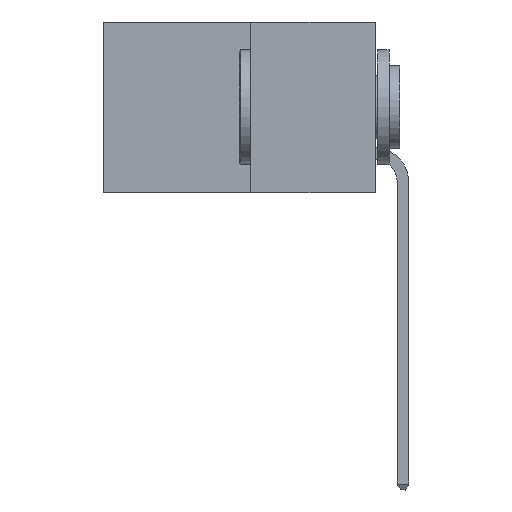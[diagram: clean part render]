
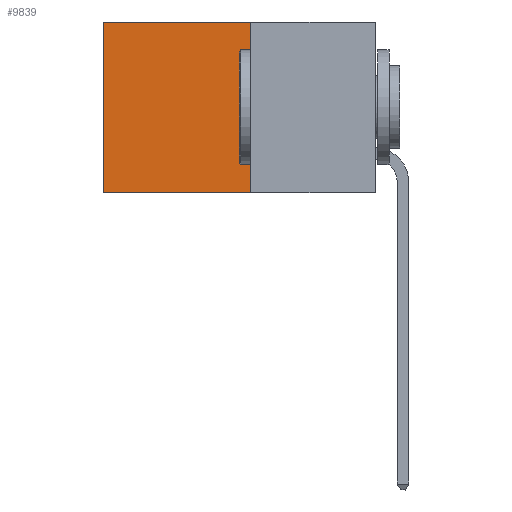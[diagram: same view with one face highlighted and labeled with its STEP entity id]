
A CAD part, left-side view. The second image highlights one B-rep face of the part: STEP entity #9839.
In plain terms, the highlighted planar face has unit normal (-1, 0, 0).
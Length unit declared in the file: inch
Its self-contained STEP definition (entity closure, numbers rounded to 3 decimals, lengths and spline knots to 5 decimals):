
#1183 = VERTEX_POINT ( 'NONE', #14891 ) ;
#7440 = CARTESIAN_POINT ( 'NONE',  ( 0.277, 0.27, 0. ) ) ;
#7531 = DIRECTION ( 'NONE',  ( 0., 1., 0. ) ) ;
#8829 = LINE ( 'NONE', #8898, #19447 ) ;
#8898 = CARTESIAN_POINT ( 'NONE',  ( 0.277, 0.59, -0.37 ) ) ;
#9678 = ORIENTED_EDGE ( 'NONE', *, *, #10059, .F. ) ;
#9839 = ADVANCED_FACE ( 'NONE', ( #27008 ), #12012, .F. ) ;
#9969 = CARTESIAN_POINT ( 'NONE',  ( 0.277, 0.27, -0.37 ) ) ;
#10059 = EDGE_CURVE ( 'NONE', #13811, #11825, #21227, .T. ) ;
#11825 = VERTEX_POINT ( 'NONE', #22484 ) ;
#12012 = PLANE ( 'NONE',  #18712 ) ;
#12119 = DIRECTION ( 'NONE',  ( 0., 1., 0. ) ) ;
#13300 = CARTESIAN_POINT ( 'NONE',  ( 0.277, 0.27, 0. ) ) ;
#13811 = VERTEX_POINT ( 'NONE', #13300 ) ;
#14052 = VECTOR ( 'NONE', #7531, 39.37008 ) ;
#14156 = LINE ( 'NONE', #9969, #25283 ) ;
#14185 = DIRECTION ( 'NONE',  ( 0., 0., -1. ) ) ;
#14630 = EDGE_CURVE ( 'NONE', #11825, #1183, #14156, .T. ) ;
#14891 = CARTESIAN_POINT ( 'NONE',  ( 0.277, 0.59, -0.37 ) ) ;
#15613 = VECTOR ( 'NONE', #23288, 39.37008 ) ;
#16370 = EDGE_CURVE ( 'NONE', #13811, #25216, #24551, .T. ) ;
#18712 = AXIS2_PLACEMENT_3D ( 'NONE', #24642, #26665, #14185 ) ;
#19447 = VECTOR ( 'NONE', #21589, 39.37008 ) ;
#19501 = EDGE_CURVE ( 'NONE', #25216, #1183, #8829, .T. ) ;
#21168 = CARTESIAN_POINT ( 'NONE',  ( 0.277, 0.27, -0.37 ) ) ;
#21227 = LINE ( 'NONE', #21168, #15613 ) ;
#21589 = DIRECTION ( 'NONE',  ( 0., 0., -1. ) ) ;
#22177 = ORIENTED_EDGE ( 'NONE', *, *, #16370, .T. ) ;
#22484 = CARTESIAN_POINT ( 'NONE',  ( 0.277, 0.27, -0.37 ) ) ;
#23288 = DIRECTION ( 'NONE',  ( 0., 0., -1. ) ) ;
#23738 = ORIENTED_EDGE ( 'NONE', *, *, #19501, .T. ) ;
#23976 = CARTESIAN_POINT ( 'NONE',  ( 0.277, 0.59, 0. ) ) ;
#24497 = EDGE_LOOP ( 'NONE', ( #23738, #26835, #9678, #22177 ) ) ;
#24551 = LINE ( 'NONE', #7440, #14052 ) ;
#24642 = CARTESIAN_POINT ( 'NONE',  ( 0.277, 0.27, -0.37 ) ) ;
#25216 = VERTEX_POINT ( 'NONE', #23976 ) ;
#25283 = VECTOR ( 'NONE', #12119, 39.37008 ) ;
#26665 = DIRECTION ( 'NONE',  ( 1., 0., 0. ) ) ;
#26835 = ORIENTED_EDGE ( 'NONE', *, *, #14630, .F. ) ;
#27008 = FACE_OUTER_BOUND ( 'NONE', #24497, .T. ) ;
